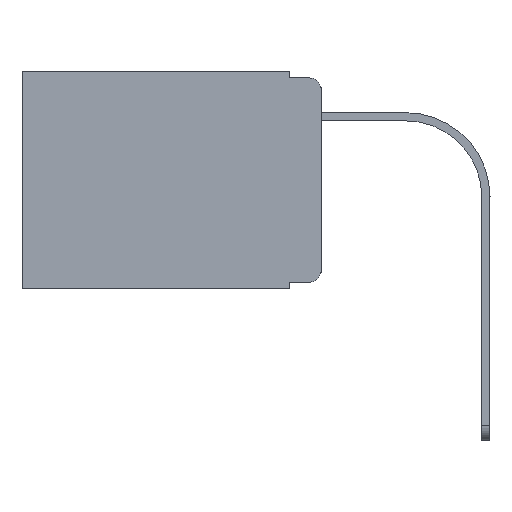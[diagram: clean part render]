
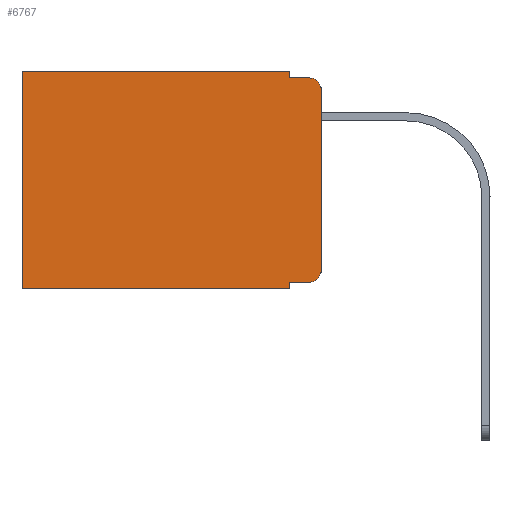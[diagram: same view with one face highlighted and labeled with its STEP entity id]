
A CAD part, left-side view. The second image highlights one B-rep face of the part: STEP entity #6767.
In plain terms, the highlighted planar face has unit normal (-1, 0, 0).
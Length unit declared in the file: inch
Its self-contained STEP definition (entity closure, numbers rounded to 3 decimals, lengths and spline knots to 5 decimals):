
#132 = ORIENTED_EDGE ( 'NONE', *, *, #23060, .T. ) ;
#146 = CARTESIAN_POINT ( 'NONE',  ( 0.298, 0.051, 0. ) ) ;
#428 = ORIENTED_EDGE ( 'NONE', *, *, #1189, .F. ) ;
#618 = AXIS2_PLACEMENT_3D ( 'NONE', #10057, #12162, #19712 ) ;
#1116 = DIRECTION ( 'NONE',  ( 1., 0., 0. ) ) ;
#1189 = EDGE_CURVE ( 'NONE', #21286, #21314, #21920, .T. ) ;
#1415 = CARTESIAN_POINT ( 'NONE',  ( 0.298, 0.02, -0.313 ) ) ;
#1452 = LINE ( 'NONE', #24441, #21016 ) ;
#1586 = DIRECTION ( 'NONE',  ( 0., 0., -1. ) ) ;
#2386 = CARTESIAN_POINT ( 'NONE',  ( 0.298, 0.051, 0. ) ) ;
#2867 = CARTESIAN_POINT ( 'NONE',  ( 0.298, 0., 0. ) ) ;
#2962 = VERTEX_POINT ( 'NONE', #11896 ) ;
#3298 = EDGE_CURVE ( 'NONE', #3315, #19108, #1452, .T. ) ;
#3315 = VERTEX_POINT ( 'NONE', #9262 ) ;
#3603 = VECTOR ( 'NONE', #14387, 39.37008 ) ;
#4112 = DIRECTION ( 'NONE',  ( 0., 0., -1. ) ) ;
#4407 = ORIENTED_EDGE ( 'NONE', *, *, #15550, .T. ) ;
#4484 = VERTEX_POINT ( 'NONE', #2386 ) ;
#4502 = EDGE_CURVE ( 'NONE', #11655, #21314, #23890, .T. ) ;
#4598 = CARTESIAN_POINT ( 'NONE',  ( 0.298, 0., 0. ) ) ;
#4878 = EDGE_CURVE ( 'NONE', #4484, #3315, #18266, .T. ) ;
#5431 = VECTOR ( 'NONE', #22959, 39.37008 ) ;
#5443 = DIRECTION ( 'NONE',  ( 0., 0., -1. ) ) ;
#5927 = LINE ( 'NONE', #15327, #18629 ) ;
#5985 = VERTEX_POINT ( 'NONE', #9599 ) ;
#6767 = ADVANCED_FACE ( 'NONE', ( #10665 ), #18320, .F. ) ;
#7220 = DIRECTION ( 'NONE',  ( 0., 0., -1. ) ) ;
#7272 = DIRECTION ( 'NONE',  ( 0., 0., -1. ) ) ;
#7370 = CIRCLE ( 'NONE', #12576, 0.02 ) ;
#7568 = VECTOR ( 'NONE', #4112, 39.37008 ) ;
#8110 = EDGE_LOOP ( 'NONE', ( #20175, #8510, #428, #12021, #21822, #11172, #11898, #15731, #132, #4407 ) ) ;
#8510 = ORIENTED_EDGE ( 'NONE', *, *, #4502, .T. ) ;
#8735 = CARTESIAN_POINT ( 'NONE',  ( 0.298, 0., -0.03 ) ) ;
#9262 = CARTESIAN_POINT ( 'NONE',  ( 0.298, 0.473, 0. ) ) ;
#9346 = EDGE_CURVE ( 'NONE', #24152, #2962, #20839, .T. ) ;
#9599 = CARTESIAN_POINT ( 'NONE',  ( 0.298, 0., -0.313 ) ) ;
#9807 = CARTESIAN_POINT ( 'NONE',  ( 0.298, 0.02, -0.01 ) ) ;
#9947 = DIRECTION ( 'NONE',  ( 0., -1., 0. ) ) ;
#10036 = CARTESIAN_POINT ( 'NONE',  ( 0.298, 0., 0. ) ) ;
#10057 = CARTESIAN_POINT ( 'NONE',  ( 0.298, 0.02, -0.03 ) ) ;
#10299 = CARTESIAN_POINT ( 'NONE',  ( 0.298, 0.051, -0.01 ) ) ;
#10602 = DIRECTION ( 'NONE',  ( -1., 0., 0. ) ) ;
#10665 = FACE_OUTER_BOUND ( 'NONE', #8110, .T. ) ;
#10829 = CARTESIAN_POINT ( 'NONE',  ( 0.298, 0., -0.343 ) ) ;
#11172 = ORIENTED_EDGE ( 'NONE', *, *, #3298, .T. ) ;
#11287 = CARTESIAN_POINT ( 'NONE',  ( 0.298, 0.051, 0. ) ) ;
#11655 = VERTEX_POINT ( 'NONE', #8735 ) ;
#11896 = CARTESIAN_POINT ( 'NONE',  ( 0.298, 0.051, -0.343 ) ) ;
#11898 = ORIENTED_EDGE ( 'NONE', *, *, #21594, .F. ) ;
#12021 = ORIENTED_EDGE ( 'NONE', *, *, #15671, .F. ) ;
#12162 = DIRECTION ( 'NONE',  ( -1., 0., 0. ) ) ;
#12576 = AXIS2_PLACEMENT_3D ( 'NONE', #1415, #10602, #7220 ) ;
#13156 = VERTEX_POINT ( 'NONE', #20648 ) ;
#13164 = AXIS2_PLACEMENT_3D ( 'NONE', #2867, #1116, #7272 ) ;
#13743 = EDGE_CURVE ( 'NONE', #11655, #5985, #23434, .T. ) ;
#14387 = DIRECTION ( 'NONE',  ( 0., -1., 0. ) ) ;
#15327 = CARTESIAN_POINT ( 'NONE',  ( 0.298, 0.051, -0.333 ) ) ;
#15550 = EDGE_CURVE ( 'NONE', #13156, #5985, #7370, .T. ) ;
#15671 = EDGE_CURVE ( 'NONE', #4484, #21286, #24643, .T. ) ;
#15731 = ORIENTED_EDGE ( 'NONE', *, *, #9346, .F. ) ;
#16136 = CARTESIAN_POINT ( 'NONE',  ( 0.298, 0.051, -0.333 ) ) ;
#18266 = LINE ( 'NONE', #10036, #21519 ) ;
#18320 = PLANE ( 'NONE',  #13164 ) ;
#18629 = VECTOR ( 'NONE', #9947, 39.37008 ) ;
#19108 = VERTEX_POINT ( 'NONE', #24167 ) ;
#19712 = DIRECTION ( 'NONE',  ( 0., 0., -1. ) ) ;
#20175 = ORIENTED_EDGE ( 'NONE', *, *, #13743, .F. ) ;
#20648 = CARTESIAN_POINT ( 'NONE',  ( 0.298, 0.02, -0.333 ) ) ;
#20839 = LINE ( 'NONE', #11287, #5431 ) ;
#21016 = VECTOR ( 'NONE', #1586, 39.37008 ) ;
#21286 = VERTEX_POINT ( 'NONE', #10299 ) ;
#21314 = VERTEX_POINT ( 'NONE', #9807 ) ;
#21401 = VECTOR ( 'NONE', #5443, 39.37008 ) ;
#21519 = VECTOR ( 'NONE', #21585, 39.37008 ) ;
#21585 = DIRECTION ( 'NONE',  ( 0., 1., 0. ) ) ;
#21594 = EDGE_CURVE ( 'NONE', #2962, #19108, #23883, .T. ) ;
#21822 = ORIENTED_EDGE ( 'NONE', *, *, #4878, .T. ) ;
#21920 = LINE ( 'NONE', #23670, #3603 ) ;
#22247 = VECTOR ( 'NONE', #22513, 39.37008 ) ;
#22513 = DIRECTION ( 'NONE',  ( 0., 1., 0. ) ) ;
#22959 = DIRECTION ( 'NONE',  ( 0., 0., -1. ) ) ;
#23060 = EDGE_CURVE ( 'NONE', #24152, #13156, #5927, .T. ) ;
#23434 = LINE ( 'NONE', #4598, #7568 ) ;
#23670 = CARTESIAN_POINT ( 'NONE',  ( 0.298, 0.051, -0.01 ) ) ;
#23883 = LINE ( 'NONE', #10829, #22247 ) ;
#23890 = CIRCLE ( 'NONE', #618, 0.02 ) ;
#24152 = VERTEX_POINT ( 'NONE', #16136 ) ;
#24167 = CARTESIAN_POINT ( 'NONE',  ( 0.298, 0.473, -0.343 ) ) ;
#24441 = CARTESIAN_POINT ( 'NONE',  ( 0.298, 0.473, 0. ) ) ;
#24643 = LINE ( 'NONE', #146, #21401 ) ;
